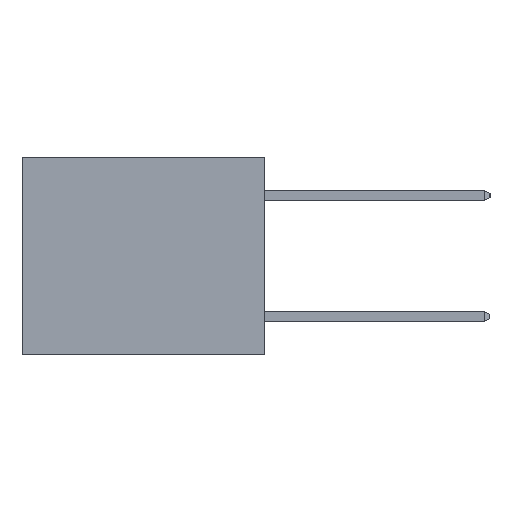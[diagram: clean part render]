
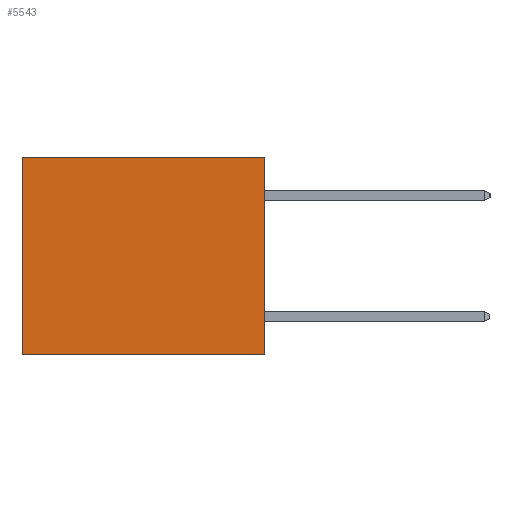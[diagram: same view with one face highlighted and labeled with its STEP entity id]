
A CAD part, left-side view. The second image highlights one B-rep face of the part: STEP entity #5543.
In plain terms, the highlighted planar face has unit normal (-1, 0, 0).
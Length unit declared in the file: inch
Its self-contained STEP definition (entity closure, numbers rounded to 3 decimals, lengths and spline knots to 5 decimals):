
#386 = DIRECTION ( 'NONE',  ( 0., 1., 0. ) ) ;
#795 = DIRECTION ( 'NONE',  ( 0., 1., 0. ) ) ;
#1023 = CARTESIAN_POINT ( 'NONE',  ( 0.3165, 0.6, -0.49 ) ) ;
#1703 = CARTESIAN_POINT ( 'NONE',  ( 0.3165, 0.6, 0. ) ) ;
#1714 = LINE ( 'NONE', #12269, #8731 ) ;
#2077 = DIRECTION ( 'NONE',  ( 0., 0., -1. ) ) ;
#2840 = VERTEX_POINT ( 'NONE', #1703 ) ;
#2963 = DIRECTION ( 'NONE',  ( 0., 0., -1. ) ) ;
#4592 = PLANE ( 'NONE',  #7437 ) ;
#4767 = DIRECTION ( 'NONE',  ( 1., 0., 0. ) ) ;
#5448 = CARTESIAN_POINT ( 'NONE',  ( 0.3165, 0., 0. ) ) ;
#5543 = ADVANCED_FACE ( 'NONE', ( #14065 ), #4592, .F. ) ;
#5820 = EDGE_CURVE ( 'NONE', #2840, #13495, #13363, .T. ) ;
#7437 = AXIS2_PLACEMENT_3D ( 'NONE', #12219, #4767, #11108 ) ;
#8421 = EDGE_CURVE ( 'NONE', #14603, #13495, #1714, .T. ) ;
#8731 = VECTOR ( 'NONE', #795, 39.37008 ) ;
#8810 = EDGE_LOOP ( 'NONE', ( #9439, #10937, #9499, #10806 ) ) ;
#9439 = ORIENTED_EDGE ( 'NONE', *, *, #5820, .T. ) ;
#9499 = ORIENTED_EDGE ( 'NONE', *, *, #11285, .F. ) ;
#9970 = VECTOR ( 'NONE', #2963, 39.37008 ) ;
#10300 = CARTESIAN_POINT ( 'NONE',  ( 0.3165, 0., -0.49 ) ) ;
#10626 = CARTESIAN_POINT ( 'NONE',  ( 0.3165, 0., 0. ) ) ;
#10806 = ORIENTED_EDGE ( 'NONE', *, *, #13534, .T. ) ;
#10937 = ORIENTED_EDGE ( 'NONE', *, *, #8421, .F. ) ;
#11108 = DIRECTION ( 'NONE',  ( 0., 0., -1. ) ) ;
#11285 = EDGE_CURVE ( 'NONE', #15435, #14603, #15789, .T. ) ;
#12219 = CARTESIAN_POINT ( 'NONE',  ( 0.3165, 0., -0.49 ) ) ;
#12269 = CARTESIAN_POINT ( 'NONE',  ( 0.3165, 0., -0.49 ) ) ;
#13243 = CARTESIAN_POINT ( 'NONE',  ( 0.3165, 0.6, -0.49 ) ) ;
#13363 = LINE ( 'NONE', #13243, #9970 ) ;
#13495 = VERTEX_POINT ( 'NONE', #1023 ) ;
#13509 = CARTESIAN_POINT ( 'NONE',  ( 0.3165, 0., -0.49 ) ) ;
#13534 = EDGE_CURVE ( 'NONE', #15435, #2840, #14669, .T. ) ;
#14065 = FACE_OUTER_BOUND ( 'NONE', #8810, .T. ) ;
#14603 = VERTEX_POINT ( 'NONE', #10300 ) ;
#14669 = LINE ( 'NONE', #5448, #14690 ) ;
#14690 = VECTOR ( 'NONE', #386, 39.37008 ) ;
#15388 = VECTOR ( 'NONE', #2077, 39.37008 ) ;
#15435 = VERTEX_POINT ( 'NONE', #10626 ) ;
#15789 = LINE ( 'NONE', #13509, #15388 ) ;
